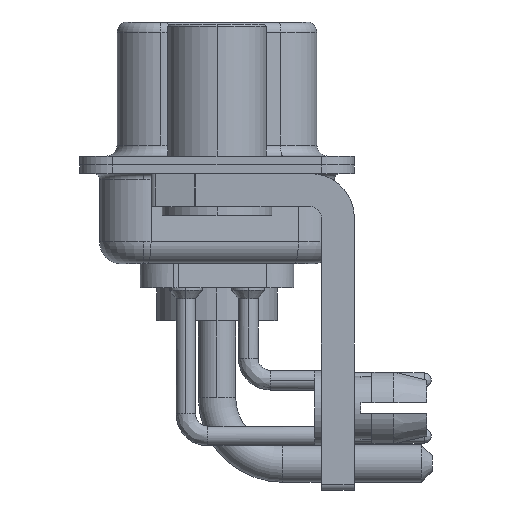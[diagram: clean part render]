
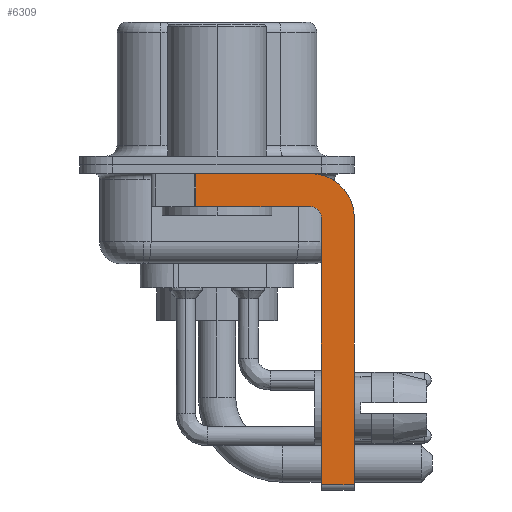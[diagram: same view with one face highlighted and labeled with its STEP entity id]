
A CAD part, left-side view. The second image highlights one B-rep face of the part: STEP entity #6309.
In plain terms, the highlighted planar face has unit normal (-1, 0, 0).
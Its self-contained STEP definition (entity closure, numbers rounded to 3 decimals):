
#441 = DIRECTION ( 'NONE',  ( 0., 0., 1. ) ) ;
#1139 = DIRECTION ( 'NONE',  ( 0., 0., 1. ) ) ;
#1187 = CARTESIAN_POINT ( 'NONE',  ( -2.9, -4.25, -14.55 ) ) ;
#1268 = CARTESIAN_POINT ( 'NONE',  ( -2.9, -4.25, -2.4 ) ) ;
#1424 = EDGE_LOOP ( 'NONE', ( #14001, #21581, #20003, #11171, #23689, #16570, #19128, #17185 ) ) ;
#1967 = DIRECTION ( 'NONE',  ( 0., -1., 0. ) ) ;
#2055 = EDGE_CURVE ( 'NONE', #6746, #5918, #16805, .T. ) ;
#2679 = VECTOR ( 'NONE', #7829, 1000. ) ;
#3472 = CARTESIAN_POINT ( 'NONE',  ( -2.9, -4.25, -1.9 ) ) ;
#3938 = VERTEX_POINT ( 'NONE', #3472 ) ;
#5393 = VERTEX_POINT ( 'NONE', #19491 ) ;
#5899 = LINE ( 'NONE', #19911, #25830 ) ;
#5918 = VERTEX_POINT ( 'NONE', #9879 ) ;
#6024 = CIRCLE ( 'NONE', #22772, 0.5 ) ;
#6309 = ADVANCED_FACE ( 'NONE', ( #17046 ), #25067, .F. ) ;
#6746 = VERTEX_POINT ( 'NONE', #25157 ) ;
#7037 = VERTEX_POINT ( 'NONE', #20271 ) ;
#7123 = EDGE_CURVE ( 'NONE', #13390, #3938, #6024, .T. ) ;
#7162 = CARTESIAN_POINT ( 'NONE',  ( -2.9, -4.75, -2.4 ) ) ;
#7378 = CARTESIAN_POINT ( 'NONE',  ( -2.9, 0.978, -1.9 ) ) ;
#7411 = DIRECTION ( 'NONE',  ( 0., 0., -1. ) ) ;
#7829 = DIRECTION ( 'NONE',  ( 0., 0., -1. ) ) ;
#7958 = EDGE_CURVE ( 'NONE', #5918, #22314, #14488, .T. ) ;
#9088 = CARTESIAN_POINT ( 'NONE',  ( -2.9, -6.25, -14.55 ) ) ;
#9850 = DIRECTION ( 'NONE',  ( 0., 0., -1. ) ) ;
#9879 = CARTESIAN_POINT ( 'NONE',  ( -2.9, -6.25, -2.4 ) ) ;
#10411 = LINE ( 'NONE', #18379, #20481 ) ;
#10714 = VERTEX_POINT ( 'NONE', #7378 ) ;
#11171 = ORIENTED_EDGE ( 'NONE', *, *, #7123, .F. ) ;
#11341 = CARTESIAN_POINT ( 'NONE',  ( -2.9, -4.25, -1.9 ) ) ;
#11750 = CARTESIAN_POINT ( 'NONE',  ( -2.9, 0.978, -1.9 ) ) ;
#11804 = AXIS2_PLACEMENT_3D ( 'NONE', #17344, #15507, #7411 ) ;
#12698 = AXIS2_PLACEMENT_3D ( 'NONE', #13253, #21235, #9850 ) ;
#13253 = CARTESIAN_POINT ( 'NONE',  ( -2.9, -4.25, -2.4 ) ) ;
#13390 = VERTEX_POINT ( 'NONE', #7162 ) ;
#14001 = ORIENTED_EDGE ( 'NONE', *, *, #25771, .F. ) ;
#14224 = CARTESIAN_POINT ( 'NONE',  ( -2.9, -6.25, -2.4 ) ) ;
#14488 = LINE ( 'NONE', #14224, #20265 ) ;
#15401 = DIRECTION ( 'NONE',  ( -1., 0., 0. ) ) ;
#15507 = DIRECTION ( 'NONE',  ( 1., 0., 0. ) ) ;
#15620 = VECTOR ( 'NONE', #20707, 1000. ) ;
#16362 = EDGE_CURVE ( 'NONE', #5393, #13390, #10411, .T. ) ;
#16570 = ORIENTED_EDGE ( 'NONE', *, *, #22767, .T. ) ;
#16805 = CIRCLE ( 'NONE', #11804, 2. ) ;
#17046 = FACE_OUTER_BOUND ( 'NONE', #1424, .T. ) ;
#17185 = ORIENTED_EDGE ( 'NONE', *, *, #2055, .F. ) ;
#17218 = LINE ( 'NONE', #11341, #20726 ) ;
#17344 = CARTESIAN_POINT ( 'NONE',  ( -2.9, -4.25, -2.4 ) ) ;
#18012 = LINE ( 'NONE', #11750, #2679 ) ;
#18379 = CARTESIAN_POINT ( 'NONE',  ( -2.9, -4.75, -14.8 ) ) ;
#19125 = LINE ( 'NONE', #1187, #15620 ) ;
#19128 = ORIENTED_EDGE ( 'NONE', *, *, #7958, .F. ) ;
#19491 = CARTESIAN_POINT ( 'NONE',  ( -2.9, -4.75, -14.55 ) ) ;
#19911 = CARTESIAN_POINT ( 'NONE',  ( -2.9, 3., -0.4 ) ) ;
#20003 = ORIENTED_EDGE ( 'NONE', *, *, #24267, .F. ) ;
#20265 = VECTOR ( 'NONE', #24329, 1000. ) ;
#20271 = CARTESIAN_POINT ( 'NONE',  ( -2.9, 0.978, -0.4 ) ) ;
#20481 = VECTOR ( 'NONE', #441, 1000. ) ;
#20707 = DIRECTION ( 'NONE',  ( 0., -1., 0. ) ) ;
#20726 = VECTOR ( 'NONE', #25238, 1000. ) ;
#21235 = DIRECTION ( 'NONE',  ( 1., 0., 0. ) ) ;
#21581 = ORIENTED_EDGE ( 'NONE', *, *, #21657, .T. ) ;
#21657 = EDGE_CURVE ( 'NONE', #7037, #10714, #18012, .T. ) ;
#22314 = VERTEX_POINT ( 'NONE', #9088 ) ;
#22767 = EDGE_CURVE ( 'NONE', #5393, #22314, #19125, .T. ) ;
#22772 = AXIS2_PLACEMENT_3D ( 'NONE', #1268, #15401, #1139 ) ;
#23689 = ORIENTED_EDGE ( 'NONE', *, *, #16362, .F. ) ;
#24267 = EDGE_CURVE ( 'NONE', #3938, #10714, #17218, .T. ) ;
#24329 = DIRECTION ( 'NONE',  ( 0., 0., -1. ) ) ;
#25067 = PLANE ( 'NONE',  #12698 ) ;
#25157 = CARTESIAN_POINT ( 'NONE',  ( -2.9, -4.25, -0.4 ) ) ;
#25238 = DIRECTION ( 'NONE',  ( 0., 1., 0. ) ) ;
#25771 = EDGE_CURVE ( 'NONE', #7037, #6746, #5899, .T. ) ;
#25830 = VECTOR ( 'NONE', #1967, 1000. ) ;
